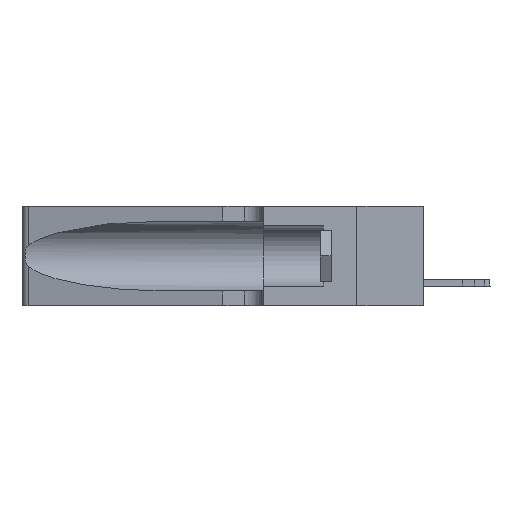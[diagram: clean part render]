
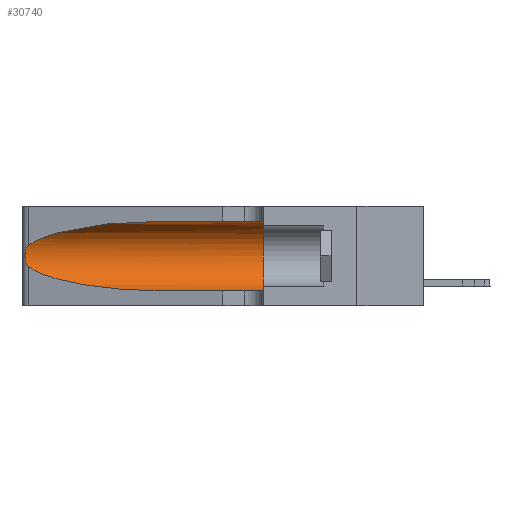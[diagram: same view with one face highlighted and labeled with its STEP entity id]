
A CAD part, left-side view. The second image highlights one B-rep face of the part: STEP entity #30740.
In plain terms, the highlighted cylindrical face has radius 3.308 mm (diameter 6.617 mm), a partial arc.
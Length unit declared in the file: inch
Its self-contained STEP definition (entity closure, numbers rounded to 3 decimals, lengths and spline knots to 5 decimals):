
#112 = CARTESIAN_POINT ( 'NONE',  ( 0.25487, 1.22718, 0.14631 ) ) ;
#157 = EDGE_LOOP ( 'NONE', ( #4482, #356, #3749, #8324, #9149, #14384 ) ) ;
#356 = ORIENTED_EDGE ( 'NONE', *, *, #15458, .T. ) ;
#914 = CARTESIAN_POINT ( 'NONE',  ( 0.26075, 1.23896, 0.19203 ) ) ;
#1095 = EDGE_CURVE ( 'NONE', #9287, #6702, #26060, .T. ) ;
#1802 = DIRECTION ( 'NONE',  ( 0., 0., 1. ) ) ;
#3749 = ORIENTED_EDGE ( 'NONE', *, *, #37543, .T. ) ;
#4436 = CARTESIAN_POINT ( 'NONE',  ( 0.25487, 1.22718, 0.22369 ) ) ;
#4482 = ORIENTED_EDGE ( 'NONE', *, *, #10335, .T. ) ;
#5036 = DIRECTION ( 'NONE',  ( 0., -1., 0. ) ) ;
#5136 = CARTESIAN_POINT ( 'NONE',  ( 0.1305, 0.72297, 0.31525 ) ) ;
#6696 = CYLINDRICAL_SURFACE ( 'NONE', #23198, 0.13025 ) ;
#6702 = VERTEX_POINT ( 'NONE', #40596 ) ;
#7226 = CARTESIAN_POINT ( 'NONE',  ( 0.25639, 1.23184, 0.21858 ) ) ;
#7785 = CARTESIAN_POINT ( 'NONE',  ( 0.25487, 1.22718, 0.14631 ) ) ;
#8079 = CARTESIAN_POINT ( 'NONE',  ( 0.25555, 1.22993, 0.14849 ) ) ;
#8288 = VECTOR ( 'NONE', #5036, 39.37008 ) ;
#8324 = ORIENTED_EDGE ( 'NONE', *, *, #36248, .T. ) ;
#9149 = ORIENTED_EDGE ( 'NONE', *, *, #11253, .F. ) ;
#9287 = VERTEX_POINT ( 'NONE', #27470 ) ;
#10335 = EDGE_CURVE ( 'NONE', #9287, #23467, #31831, .T. ) ;
#11253 = EDGE_CURVE ( 'NONE', #6702, #16737, #18118, .T. ) ;
#11842 = DIRECTION ( 'NONE',  ( 0., 1., 0. ) ) ;
#13097 = VECTOR ( 'NONE', #31466, 39.37008 ) ;
#13570 = CARTESIAN_POINT ( 'NONE',  ( 0.25555, 1.22994, 0.2215 ) ) ;
#14146 = CARTESIAN_POINT ( 'NONE',  ( 0.25856, 1.23593, 0.16098 ) ) ;
#14384 = ORIENTED_EDGE ( 'NONE', *, *, #1095, .F. ) ;
#15288 = B_SPLINE_CURVE_WITH_KNOTS ( 'NONE', 3,
 ( #4436, #13570, #7226, #38930, #19974, #16880, #914, #23125, #26305, #14146, #20537, #30046, #8079, #7785 ),
 .UNSPECIFIED., .F., .F.,
 ( 4, 2, 2, 2, 2, 2, 4 ),
 ( 0., 0.00027, 0.00053, 0.00107, 0.0016, 0.00187, 0.00214 ),
 .UNSPECIFIED. ) ;
#15458 = EDGE_CURVE ( 'NONE', #23467, #32019, #15288, .T. ) ;
#15946 = CARTESIAN_POINT ( 'NONE',  ( 0.2373, 1.15595, 0.08982 ) ) ;
#16737 = VERTEX_POINT ( 'NONE', #29103 ) ;
#16880 = CARTESIAN_POINT ( 'NONE',  ( 0.26018, 1.23835, 0.19895 ) ) ;
#17109 = AXIS2_PLACEMENT_3D ( 'NONE', #30813, #11842, #1802 ) ;
#18118 = CIRCLE ( 'NONE', #17109, 0.13025 ) ;
#19974 = CARTESIAN_POINT ( 'NONE',  ( 0.25854, 1.2359, 0.20912 ) ) ;
#20537 = CARTESIAN_POINT ( 'NONE',  ( 0.25789, 1.23486, 0.15765 ) ) ;
#21188 = CARTESIAN_POINT ( 'NONE',  ( 0.1305, 1.61858, 0.185 ) ) ;
#23125 = CARTESIAN_POINT ( 'NONE',  ( 0.26075, 1.23896, 0.178 ) ) ;
#23198 = AXIS2_PLACEMENT_3D ( 'NONE', #21188, #40583, #40315 ) ;
#23467 = VERTEX_POINT ( 'NONE', #32326 ) ;
#24633 = CARTESIAN_POINT ( 'NONE',  ( 0.18966, 0.96281, 0.31525 ) ) ;
#25308 = VERTEX_POINT ( 'NONE', #25897 ) ;
#25897 = CARTESIAN_POINT ( 'NONE',  ( 0.1305, 0.72297, 0.05475 ) ) ;
#26060 = LINE ( 'NONE', #39382, #8288 ) ;
#26305 = CARTESIAN_POINT ( 'NONE',  ( 0.26017, 1.23833, 0.17102 ) ) ;
#27224 = CARTESIAN_POINT ( 'NONE',  ( 0.2373, 1.15595, 0.28018 ) ) ;
#27470 = CARTESIAN_POINT ( 'NONE',  ( 0.1305, 0.72297, 0.31525 ) ) ;
#29103 = CARTESIAN_POINT ( 'NONE',  ( 0.1305, 0.35, 0.05475 ) ) ;
#29985 =( BOUNDED_CURVE ( )  B_SPLINE_CURVE ( 3, ( #112, #15946, #34966, #40929 ),
 .UNSPECIFIED., .F., .F. ) 
 B_SPLINE_CURVE_WITH_KNOTS ( ( 4, 4 ),
 ( 3.44316, 4.71239 ),
 .UNSPECIFIED. ) 
 CURVE ( )  GEOMETRIC_REPRESENTATION_ITEM ( )  RATIONAL_B_SPLINE_CURVE ( ( 1., 0.87, 0.87, 1. ) ) 
 REPRESENTATION_ITEM ( '' )  );
#30046 = CARTESIAN_POINT ( 'NONE',  ( 0.25639, 1.23186, 0.15144 ) ) ;
#30740 = ADVANCED_FACE ( 'NONE', ( #30987 ), #6696, .F. ) ;
#30813 = CARTESIAN_POINT ( 'NONE',  ( 0.1305, 0.35, 0.185 ) ) ;
#30985 = LINE ( 'NONE', #40481, #13097 ) ;
#30987 = FACE_OUTER_BOUND ( 'NONE', #157, .T. ) ;
#31466 = DIRECTION ( 'NONE',  ( 0., -1., 0. ) ) ;
#31831 =( BOUNDED_CURVE ( )  B_SPLINE_CURVE ( 3, ( #5136, #24633, #27224, #37395 ),
 .UNSPECIFIED., .F., .T. ) 
 B_SPLINE_CURVE_WITH_KNOTS ( ( 4, 4 ),
 ( 1.5708, 2.84003 ),
 .UNSPECIFIED. ) 
 CURVE ( )  GEOMETRIC_REPRESENTATION_ITEM ( )  RATIONAL_B_SPLINE_CURVE ( ( 1., 0.87, 0.87, 1. ) ) 
 REPRESENTATION_ITEM ( '' )  );
#32019 = VERTEX_POINT ( 'NONE', #40505 ) ;
#32326 = CARTESIAN_POINT ( 'NONE',  ( 0.25487, 1.22718, 0.22369 ) ) ;
#34966 = CARTESIAN_POINT ( 'NONE',  ( 0.18966, 0.96281, 0.05475 ) ) ;
#36248 = EDGE_CURVE ( 'NONE', #25308, #16737, #30985, .T. ) ;
#37395 = CARTESIAN_POINT ( 'NONE',  ( 0.25487, 1.22718, 0.22369 ) ) ;
#37543 = EDGE_CURVE ( 'NONE', #32019, #25308, #29985, .T. ) ;
#38930 = CARTESIAN_POINT ( 'NONE',  ( 0.25787, 1.23484, 0.2124 ) ) ;
#39382 = CARTESIAN_POINT ( 'NONE',  ( 0.1305, 1.61858, 0.31525 ) ) ;
#40315 = DIRECTION ( 'NONE',  ( 0., 0., -1. ) ) ;
#40481 = CARTESIAN_POINT ( 'NONE',  ( 0.1305, 1.61858, 0.05475 ) ) ;
#40505 = CARTESIAN_POINT ( 'NONE',  ( 0.25487, 1.22718, 0.14631 ) ) ;
#40583 = DIRECTION ( 'NONE',  ( 0., -1., 0. ) ) ;
#40596 = CARTESIAN_POINT ( 'NONE',  ( 0.1305, 0.35, 0.31525 ) ) ;
#40929 = CARTESIAN_POINT ( 'NONE',  ( 0.1305, 0.72297, 0.05475 ) ) ;
